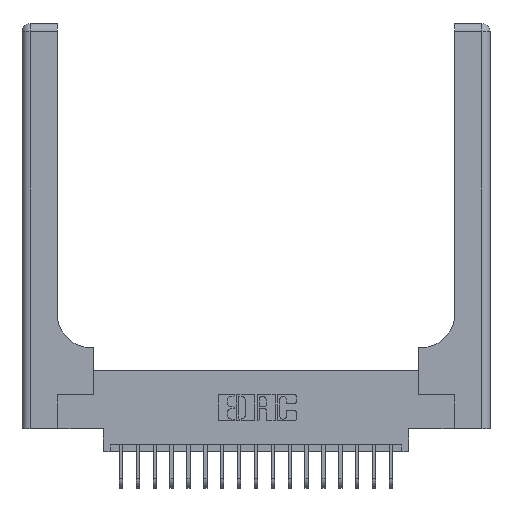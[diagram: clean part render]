
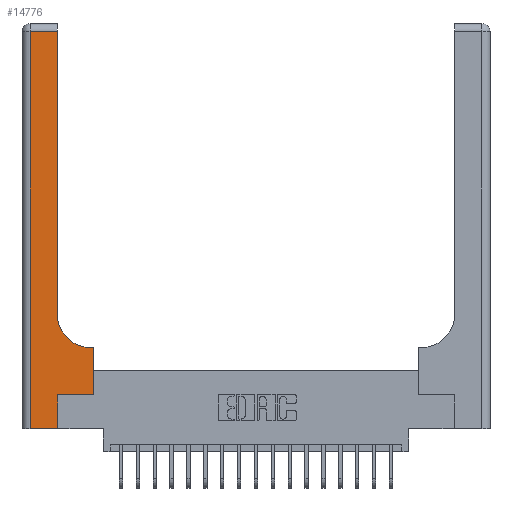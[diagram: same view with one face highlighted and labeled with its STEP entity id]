
A CAD part, top view. The second image highlights one B-rep face of the part: STEP entity #14776.
In plain terms, the highlighted planar face has unit normal (0, 0, 1).
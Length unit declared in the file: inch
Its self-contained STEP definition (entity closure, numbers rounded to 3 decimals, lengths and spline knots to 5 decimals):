
#352 = AXIS2_PLACEMENT_3D ( 'NONE', #15811, #9034, #6356 ) ;
#387 = CARTESIAN_POINT ( 'NONE',  ( 0.26, 2.94, 0.37 ) ) ;
#584 = CARTESIAN_POINT ( 'NONE',  ( 0.528, 0.25, 0.37 ) ) ;
#719 = AXIS2_PLACEMENT_3D ( 'NONE', #7152, #13716, #16930 ) ;
#1339 = DIRECTION ( 'NONE',  ( 0., -1., 0. ) ) ;
#1453 = VERTEX_POINT ( 'NONE', #15320 ) ;
#1748 = CARTESIAN_POINT ( 'NONE',  ( 0.26, 3., 0.37 ) ) ;
#2239 = PLANE ( 'NONE',  #352 ) ;
#2303 = DIRECTION ( 'NONE',  ( 1., 0., 0. ) ) ;
#2632 = VERTEX_POINT ( 'NONE', #15001 ) ;
#2677 = EDGE_CURVE ( 'NONE', #8016, #1453, #18779, .T. ) ;
#2843 = VECTOR ( 'NONE', #19723, 39.37008 ) ;
#3031 = LINE ( 'NONE', #4593, #12553 ) ;
#3848 = DIRECTION ( 'NONE',  ( 0., 1., 0. ) ) ;
#4465 = LINE ( 'NONE', #7920, #21473 ) ;
#4513 = DIRECTION ( 'NONE',  ( 1., 0., 0. ) ) ;
#4593 = CARTESIAN_POINT ( 'NONE',  ( 0., 2.94, 0.37 ) ) ;
#4764 = VERTEX_POINT ( 'NONE', #11621 ) ;
#4950 = ORIENTED_EDGE ( 'NONE', *, *, #18489, .T. ) ;
#5076 = CARTESIAN_POINT ( 'NONE',  ( 0.06, 0., 0.37 ) ) ;
#5111 = CARTESIAN_POINT ( 'NONE',  ( 0.51, 0.6, 0.37 ) ) ;
#5582 = FACE_OUTER_BOUND ( 'NONE', #7296, .T. ) ;
#5671 = VERTEX_POINT ( 'NONE', #17879 ) ;
#5735 = ORIENTED_EDGE ( 'NONE', *, *, #19653, .T. ) ;
#6190 = CARTESIAN_POINT ( 'NONE',  ( 0.265, 0.25, 0.37 ) ) ;
#6356 = DIRECTION ( 'NONE',  ( -1., 0., 0. ) ) ;
#6384 = ORIENTED_EDGE ( 'NONE', *, *, #19002, .T. ) ;
#6432 = VECTOR ( 'NONE', #3848, 39.37008 ) ;
#6462 = LINE ( 'NONE', #16473, #7860 ) ;
#7144 = VERTEX_POINT ( 'NONE', #387 ) ;
#7152 = CARTESIAN_POINT ( 'NONE',  ( 0.51, 0.85, 0.37 ) ) ;
#7296 = EDGE_LOOP ( 'NONE', ( #5735, #12065, #8188, #16005, #9995, #21689, #4950, #6384, #16423 ) ) ;
#7860 = VECTOR ( 'NONE', #1339, 39.37008 ) ;
#7920 = CARTESIAN_POINT ( 'NONE',  ( 0.26, 0.6, 0.37 ) ) ;
#8016 = VERTEX_POINT ( 'NONE', #5076 ) ;
#8188 = ORIENTED_EDGE ( 'NONE', *, *, #21042, .T. ) ;
#8989 = CARTESIAN_POINT ( 'NONE',  ( 0., 0., 0.37 ) ) ;
#9034 = DIRECTION ( 'NONE',  ( 0., 0., -1. ) ) ;
#9995 = ORIENTED_EDGE ( 'NONE', *, *, #20287, .T. ) ;
#11621 = CARTESIAN_POINT ( 'NONE',  ( 0.528, 0.25, 0.37 ) ) ;
#11927 = CARTESIAN_POINT ( 'NONE',  ( 0.26, 0.85, 0.37 ) ) ;
#11975 = LINE ( 'NONE', #1748, #6432 ) ;
#12065 = ORIENTED_EDGE ( 'NONE', *, *, #17662, .T. ) ;
#12553 = VECTOR ( 'NONE', #18160, 39.37008 ) ;
#12593 = CARTESIAN_POINT ( 'NONE',  ( 0.265, 0., 0.37 ) ) ;
#12697 = DIRECTION ( 'NONE',  ( -1., 0., 0. ) ) ;
#13716 = DIRECTION ( 'NONE',  ( 0., 0., -1. ) ) ;
#14225 = CIRCLE ( 'NONE', #719, 0.25 ) ;
#14535 = VERTEX_POINT ( 'NONE', #11927 ) ;
#14582 = EDGE_CURVE ( 'NONE', #20345, #14535, #14225, .T. ) ;
#14776 = ADVANCED_FACE ( 'NONE', ( #5582 ), #2239, .F. ) ;
#15001 = CARTESIAN_POINT ( 'NONE',  ( 0.528, 0.6, 0.37 ) ) ;
#15067 = LINE ( 'NONE', #584, #18605 ) ;
#15320 = CARTESIAN_POINT ( 'NONE',  ( 0.265, 0., 0.37 ) ) ;
#15604 = DIRECTION ( 'NONE',  ( 0., 1., 0. ) ) ;
#15811 = CARTESIAN_POINT ( 'NONE',  ( 0., 3., 0.37 ) ) ;
#16005 = ORIENTED_EDGE ( 'NONE', *, *, #2677, .T. ) ;
#16017 = VERTEX_POINT ( 'NONE', #18580 ) ;
#16423 = ORIENTED_EDGE ( 'NONE', *, *, #14582, .T. ) ;
#16472 = LINE ( 'NONE', #12593, #2843 ) ;
#16473 = CARTESIAN_POINT ( 'NONE',  ( 0.06, 3., 0.37 ) ) ;
#16764 = VECTOR ( 'NONE', #2303, 39.37008 ) ;
#16930 = DIRECTION ( 'NONE',  ( 1., 0., 0. ) ) ;
#17086 = EDGE_CURVE ( 'NONE', #5671, #4764, #21432, .T. ) ;
#17662 = EDGE_CURVE ( 'NONE', #7144, #16017, #3031, .T. ) ;
#17879 = CARTESIAN_POINT ( 'NONE',  ( 0.265, 0.25, 0.37 ) ) ;
#18160 = DIRECTION ( 'NONE',  ( -1., 0., 0. ) ) ;
#18489 = EDGE_CURVE ( 'NONE', #4764, #2632, #15067, .T. ) ;
#18580 = CARTESIAN_POINT ( 'NONE',  ( 0.06, 2.94, 0.37 ) ) ;
#18605 = VECTOR ( 'NONE', #15604, 39.37008 ) ;
#18779 = LINE ( 'NONE', #8989, #16764 ) ;
#19002 = EDGE_CURVE ( 'NONE', #2632, #20345, #4465, .T. ) ;
#19653 = EDGE_CURVE ( 'NONE', #14535, #7144, #11975, .T. ) ;
#19723 = DIRECTION ( 'NONE',  ( 0., 1., 0. ) ) ;
#20287 = EDGE_CURVE ( 'NONE', #1453, #5671, #16472, .T. ) ;
#20345 = VERTEX_POINT ( 'NONE', #5111 ) ;
#20709 = VECTOR ( 'NONE', #4513, 39.37008 ) ;
#21042 = EDGE_CURVE ( 'NONE', #16017, #8016, #6462, .T. ) ;
#21432 = LINE ( 'NONE', #6190, #20709 ) ;
#21473 = VECTOR ( 'NONE', #12697, 39.37008 ) ;
#21689 = ORIENTED_EDGE ( 'NONE', *, *, #17086, .T. ) ;
